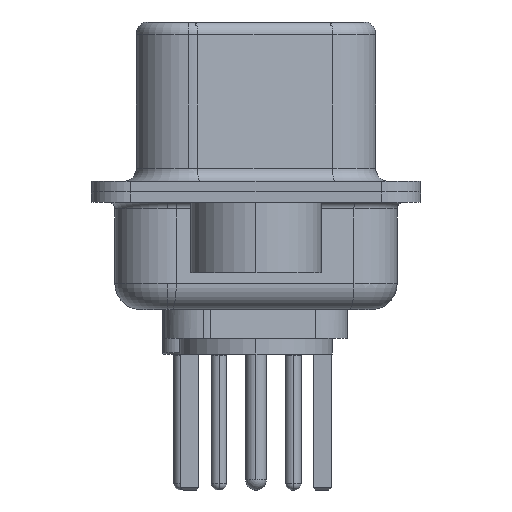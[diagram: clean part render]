
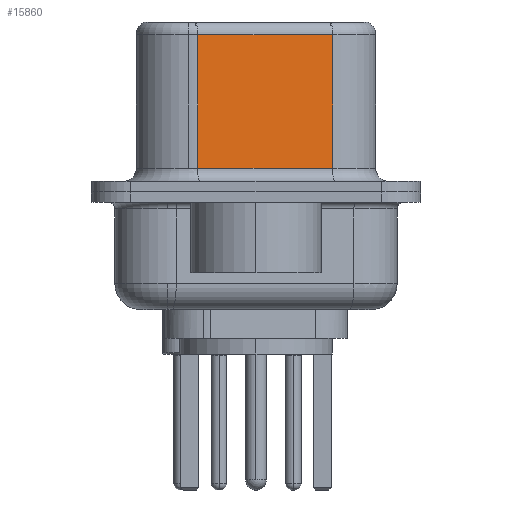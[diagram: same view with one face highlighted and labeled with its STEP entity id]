
A CAD part, left-side view. The second image highlights one B-rep face of the part: STEP entity #15860.
In plain terms, the highlighted planar face has unit normal (-0.985, -0.174, 0).
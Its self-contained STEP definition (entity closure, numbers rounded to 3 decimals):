
#248 = EDGE_CURVE ( 'NONE', #10418, #8095, #5654, .T. ) ;
#701 = ORIENTED_EDGE ( 'NONE', *, *, #10995, .T. ) ;
#908 = VECTOR ( 'NONE', #15185, 1000. ) ;
#1164 = ORIENTED_EDGE ( 'NONE', *, *, #248, .T. ) ;
#1476 = ORIENTED_EDGE ( 'NONE', *, *, #19698, .F. ) ;
#1628 = CARTESIAN_POINT ( 'NONE',  ( 3.67, 2.233, 6.02 ) ) ;
#1831 = DIRECTION ( 'NONE',  ( 0.985, 0.174, 0. ) ) ;
#3096 = DIRECTION ( 'NONE',  ( 0.174, -0.985, 0. ) ) ;
#5141 = LINE ( 'NONE', #13092, #13911 ) ;
#5654 = LINE ( 'NONE', #13428, #908 ) ;
#7610 = ORIENTED_EDGE ( 'NONE', *, *, #13899, .T. ) ;
#7944 = DIRECTION ( 'NONE',  ( -0.174, 0.985, 0. ) ) ;
#8095 = VERTEX_POINT ( 'NONE', #15155 ) ;
#9113 = VECTOR ( 'NONE', #3096, 1000. ) ;
#9175 = VECTOR ( 'NONE', #13966, 1000. ) ;
#9596 = FACE_OUTER_BOUND ( 'NONE', #15020, .T. ) ;
#10087 = CARTESIAN_POINT ( 'NONE',  ( 4.58, -2.927, 0.9 ) ) ;
#10320 = PLANE ( 'NONE',  #22488 ) ;
#10418 = VERTEX_POINT ( 'NONE', #1628 ) ;
#10549 = CARTESIAN_POINT ( 'NONE',  ( 4.58, -2.927, 6.52 ) ) ;
#10995 = EDGE_CURVE ( 'NONE', #8095, #16628, #14297, .T. ) ;
#13092 = CARTESIAN_POINT ( 'NONE',  ( 4.58, -2.927, 6.02 ) ) ;
#13428 = CARTESIAN_POINT ( 'NONE',  ( 3.67, 2.233, 6.52 ) ) ;
#13899 = EDGE_CURVE ( 'NONE', #21361, #10418, #5141, .T. ) ;
#13911 = VECTOR ( 'NONE', #7944, 1000. ) ;
#13966 = DIRECTION ( 'NONE',  ( 0., 0., -1. ) ) ;
#14131 = DIRECTION ( 'NONE',  ( -0.174, 0.985, 0. ) ) ;
#14297 = LINE ( 'NONE', #10087, #9113 ) ;
#15020 = EDGE_LOOP ( 'NONE', ( #1476, #7610, #1164, #701 ) ) ;
#15155 = CARTESIAN_POINT ( 'NONE',  ( 3.67, 2.233, 0.9 ) ) ;
#15185 = DIRECTION ( 'NONE',  ( 0., 0., -1. ) ) ;
#15860 = ADVANCED_FACE ( 'NONE', ( #9596 ), #10320, .F. ) ;
#16628 = VERTEX_POINT ( 'NONE', #21247 ) ;
#18495 = LINE ( 'NONE', #10549, #9175 ) ;
#19698 = EDGE_CURVE ( 'NONE', #21361, #16628, #18495, .T. ) ;
#21247 = CARTESIAN_POINT ( 'NONE',  ( 4.58, -2.927, 0.9 ) ) ;
#21361 = VERTEX_POINT ( 'NONE', #22025 ) ;
#22025 = CARTESIAN_POINT ( 'NONE',  ( 4.58, -2.927, 6.02 ) ) ;
#22488 = AXIS2_PLACEMENT_3D ( 'NONE', #22627, #1831, #14131 ) ;
#22627 = CARTESIAN_POINT ( 'NONE',  ( 4.58, -2.927, 6.52 ) ) ;
